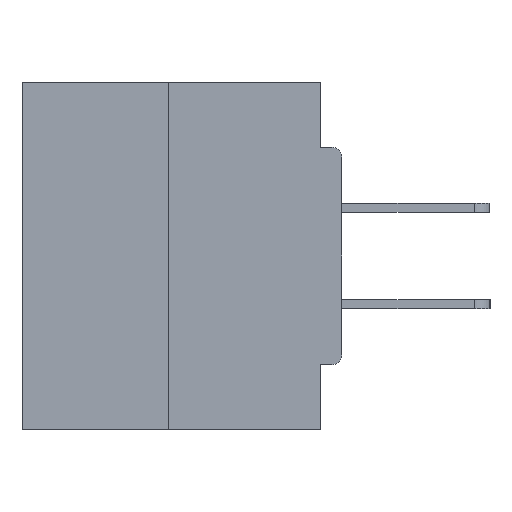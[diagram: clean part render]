
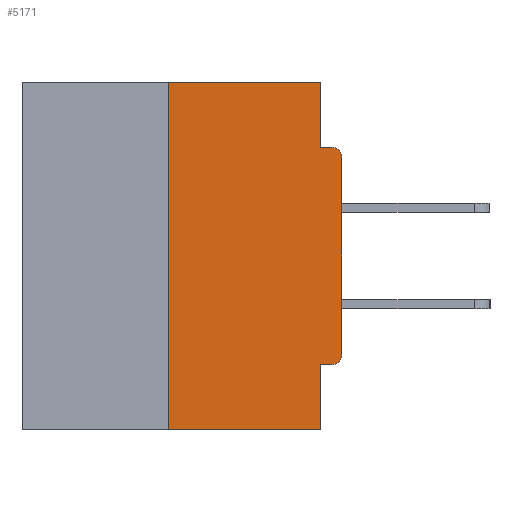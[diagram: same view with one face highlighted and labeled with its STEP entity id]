
A CAD part, left-side view. The second image highlights one B-rep face of the part: STEP entity #5171.
In plain terms, the highlighted planar face has unit normal (-1, 0, 0).
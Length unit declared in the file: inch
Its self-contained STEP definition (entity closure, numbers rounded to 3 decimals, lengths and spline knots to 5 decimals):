
#369 = EDGE_CURVE ( 'NONE', #9946, #25397, #35738, .T. ) ;
#842 = CARTESIAN_POINT ( 'NONE',  ( 0., 0.031, -0.4065 ) ) ;
#1059 = LINE ( 'NONE', #20035, #29440 ) ;
#1292 = AXIS2_PLACEMENT_3D ( 'NONE', #35823, #19084, #13560 ) ;
#2317 = LINE ( 'NONE', #10083, #31157 ) ;
#2689 = CARTESIAN_POINT ( 'NONE',  ( 0., 0., -0.3915 ) ) ;
#3364 = CARTESIAN_POINT ( 'NONE',  ( 0., 0.015, -0.3915 ) ) ;
#4560 = VECTOR ( 'NONE', #30585, 39.37008 ) ;
#5078 = LINE ( 'NONE', #23406, #32560 ) ;
#5171 = ADVANCED_FACE ( 'NONE', ( #22027 ), #35699, .F. ) ;
#5423 = DIRECTION ( 'NONE',  ( 0., 0., -1. ) ) ;
#5648 = CIRCLE ( 'NONE', #11481, 0.015 ) ;
#7414 = LINE ( 'NONE', #22960, #15293 ) ;
#8035 = VERTEX_POINT ( 'NONE', #842 ) ;
#8889 = VERTEX_POINT ( 'NONE', #33183 ) ;
#9335 = ORIENTED_EDGE ( 'NONE', *, *, #33937, .F. ) ;
#9590 = ORIENTED_EDGE ( 'NONE', *, *, #25297, .F. ) ;
#9946 = VERTEX_POINT ( 'NONE', #30907 ) ;
#10083 = CARTESIAN_POINT ( 'NONE',  ( 0., 0.25, 0. ) ) ;
#10159 = EDGE_LOOP ( 'NONE', ( #9590, #18692, #33341, #28572, #14439, #11500, #22857, #11004, #27615, #9335 ) ) ;
#10202 = VECTOR ( 'NONE', #23708, 39.37008 ) ;
#11004 = ORIENTED_EDGE ( 'NONE', *, *, #18478, .T. ) ;
#11481 = AXIS2_PLACEMENT_3D ( 'NONE', #3364, #22605, #20174 ) ;
#11500 = ORIENTED_EDGE ( 'NONE', *, *, #16810, .T. ) ;
#11677 = EDGE_CURVE ( 'NONE', #8035, #16529, #32197, .T. ) ;
#12209 = DIRECTION ( 'NONE',  ( 0., 0., 1. ) ) ;
#12532 = VECTOR ( 'NONE', #5423, 39.37008 ) ;
#13560 = DIRECTION ( 'NONE',  ( 0., 0., -1. ) ) ;
#13575 = CARTESIAN_POINT ( 'NONE',  ( 0., 0.031, 0. ) ) ;
#13868 = CARTESIAN_POINT ( 'NONE',  ( 0., 0.031, -0.5 ) ) ;
#14224 = DIRECTION ( 'NONE',  ( 0., 0., -1. ) ) ;
#14439 = ORIENTED_EDGE ( 'NONE', *, *, #17647, .F. ) ;
#15293 = VECTOR ( 'NONE', #23087, 39.37008 ) ;
#15384 = VERTEX_POINT ( 'NONE', #13575 ) ;
#15670 = DIRECTION ( 'NONE',  ( 0., 0., 1. ) ) ;
#15748 = CARTESIAN_POINT ( 'NONE',  ( 0., 0.25, 0. ) ) ;
#16256 = CARTESIAN_POINT ( 'NONE',  ( 0., 0.031, -0.5 ) ) ;
#16529 = VERTEX_POINT ( 'NONE', #13868 ) ;
#16810 = EDGE_CURVE ( 'NONE', #19779, #26087, #5648, .T. ) ;
#17114 = CIRCLE ( 'NONE', #33235, 0.015 ) ;
#17647 = EDGE_CURVE ( 'NONE', #19779, #8035, #27199, .T. ) ;
#18175 = CARTESIAN_POINT ( 'NONE',  ( 0., 0.25, -0.5 ) ) ;
#18271 = VECTOR ( 'NONE', #35607, 39.37008 ) ;
#18478 = EDGE_CURVE ( 'NONE', #8889, #25397, #17114, .T. ) ;
#18692 = ORIENTED_EDGE ( 'NONE', *, *, #25733, .F. ) ;
#18755 = CARTESIAN_POINT ( 'NONE',  ( 0., 0., -0.0935 ) ) ;
#19084 = DIRECTION ( 'NONE',  ( 1., 0., 0. ) ) ;
#19085 = VERTEX_POINT ( 'NONE', #15748 ) ;
#19779 = VERTEX_POINT ( 'NONE', #35692 ) ;
#20035 = CARTESIAN_POINT ( 'NONE',  ( 0., 0.031, 0. ) ) ;
#20174 = DIRECTION ( 'NONE',  ( 0., 0., -1. ) ) ;
#20201 = CARTESIAN_POINT ( 'NONE',  ( 0., 0.015, -0.0935 ) ) ;
#20453 = EDGE_CURVE ( 'NONE', #31610, #16529, #7414, .T. ) ;
#22027 = FACE_OUTER_BOUND ( 'NONE', #10159, .T. ) ;
#22605 = DIRECTION ( 'NONE',  ( -1., 0., 0. ) ) ;
#22857 = ORIENTED_EDGE ( 'NONE', *, *, #24314, .T. ) ;
#22960 = CARTESIAN_POINT ( 'NONE',  ( 0., 0.46, -0.5 ) ) ;
#23087 = DIRECTION ( 'NONE',  ( 0., -1., 0. ) ) ;
#23406 = CARTESIAN_POINT ( 'NONE',  ( 0., 0., 0. ) ) ;
#23708 = DIRECTION ( 'NONE',  ( 0., 1., 0. ) ) ;
#24314 = EDGE_CURVE ( 'NONE', #26087, #8889, #5078, .T. ) ;
#24944 = CARTESIAN_POINT ( 'NONE',  ( 0., 0.46, 0. ) ) ;
#25297 = EDGE_CURVE ( 'NONE', #19085, #15384, #35124, .T. ) ;
#25397 = VERTEX_POINT ( 'NONE', #20201 ) ;
#25733 = EDGE_CURVE ( 'NONE', #31610, #19085, #2317, .T. ) ;
#26043 = CARTESIAN_POINT ( 'NONE',  ( 0., 0., -0.4065 ) ) ;
#26087 = VERTEX_POINT ( 'NONE', #2689 ) ;
#27199 = LINE ( 'NONE', #26043, #10202 ) ;
#27615 = ORIENTED_EDGE ( 'NONE', *, *, #369, .F. ) ;
#28572 = ORIENTED_EDGE ( 'NONE', *, *, #11677, .F. ) ;
#29440 = VECTOR ( 'NONE', #30779, 39.37008 ) ;
#30585 = DIRECTION ( 'NONE',  ( 0., -1., 0. ) ) ;
#30779 = DIRECTION ( 'NONE',  ( 0., 0., -1. ) ) ;
#30907 = CARTESIAN_POINT ( 'NONE',  ( 0., 0.031, -0.0935 ) ) ;
#30967 = DIRECTION ( 'NONE',  ( -1., 0., 0. ) ) ;
#31157 = VECTOR ( 'NONE', #15670, 39.37008 ) ;
#31610 = VERTEX_POINT ( 'NONE', #18175 ) ;
#32197 = LINE ( 'NONE', #16256, #12532 ) ;
#32560 = VECTOR ( 'NONE', #12209, 39.37008 ) ;
#33183 = CARTESIAN_POINT ( 'NONE',  ( 0., 0., -0.1085 ) ) ;
#33235 = AXIS2_PLACEMENT_3D ( 'NONE', #33670, #30967, #14224 ) ;
#33341 = ORIENTED_EDGE ( 'NONE', *, *, #20453, .T. ) ;
#33670 = CARTESIAN_POINT ( 'NONE',  ( 0., 0.015, -0.1085 ) ) ;
#33937 = EDGE_CURVE ( 'NONE', #15384, #9946, #1059, .T. ) ;
#35124 = LINE ( 'NONE', #24944, #4560 ) ;
#35607 = DIRECTION ( 'NONE',  ( 0., -1., 0. ) ) ;
#35692 = CARTESIAN_POINT ( 'NONE',  ( 0., 0.015, -0.4065 ) ) ;
#35699 = PLANE ( 'NONE',  #1292 ) ;
#35738 = LINE ( 'NONE', #18755, #18271 ) ;
#35823 = CARTESIAN_POINT ( 'NONE',  ( 0., 0.46, 0. ) ) ;
